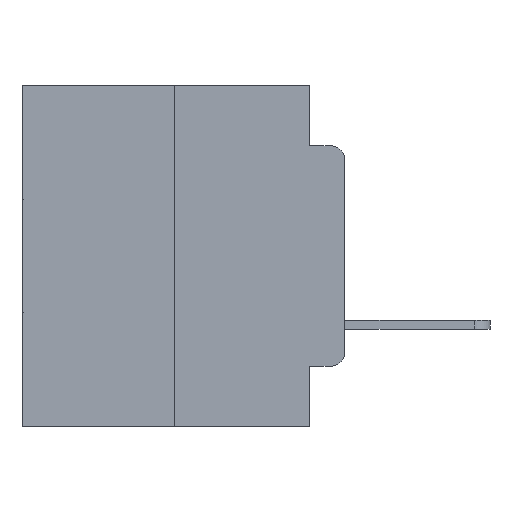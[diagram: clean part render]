
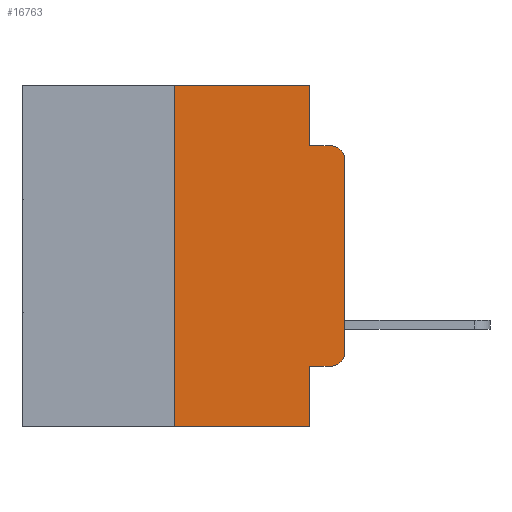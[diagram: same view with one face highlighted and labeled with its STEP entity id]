
A CAD part, left-side view. The second image highlights one B-rep face of the part: STEP entity #16763.
In plain terms, the highlighted planar face has unit normal (-1, 0, 0).
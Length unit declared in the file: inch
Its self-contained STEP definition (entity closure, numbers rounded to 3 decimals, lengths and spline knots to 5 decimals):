
#616 = DIRECTION ( 'NONE',  ( 1., 0., 0. ) ) ;
#1501 = DIRECTION ( 'NONE',  ( 0., 0., -1. ) ) ;
#1969 = VERTEX_POINT ( 'NONE', #9415 ) ;
#2576 = CARTESIAN_POINT ( 'NONE',  ( 0., 0., -0.1085 ) ) ;
#2963 = CARTESIAN_POINT ( 'NONE',  ( 0., 0.473, 0. ) ) ;
#3469 = VERTEX_POINT ( 'NONE', #17438 ) ;
#4350 = DIRECTION ( 'NONE',  ( 0., 0., 1. ) ) ;
#4463 = DIRECTION ( 'NONE',  ( 0., 0., 1. ) ) ;
#5062 = EDGE_CURVE ( 'NONE', #19786, #3469, #8488, .T. ) ;
#5736 = ORIENTED_EDGE ( 'NONE', *, *, #23668, .T. ) ;
#6091 = VECTOR ( 'NONE', #17724, 39.37008 ) ;
#6179 = EDGE_CURVE ( 'NONE', #1969, #26335, #27511, .T. ) ;
#6511 = DIRECTION ( 'NONE',  ( 0., -1., 0. ) ) ;
#6670 = VECTOR ( 'NONE', #14076, 39.37008 ) ;
#6709 = CARTESIAN_POINT ( 'NONE',  ( 0., 0.25, 0. ) ) ;
#6812 = LINE ( 'NONE', #9000, #6091 ) ;
#6977 = CARTESIAN_POINT ( 'NONE',  ( 0., 0., -0.3915 ) ) ;
#7083 = CARTESIAN_POINT ( 'NONE',  ( 0., 0.25, -0.5 ) ) ;
#7848 = ORIENTED_EDGE ( 'NONE', *, *, #14998, .F. ) ;
#7859 = CARTESIAN_POINT ( 'NONE',  ( 0., 0.051, 0. ) ) ;
#8178 = ORIENTED_EDGE ( 'NONE', *, *, #5062, .T. ) ;
#8261 = CARTESIAN_POINT ( 'NONE',  ( 0., 0.473, 0. ) ) ;
#8488 = LINE ( 'NONE', #9616, #19468 ) ;
#8993 = CIRCLE ( 'NONE', #9815, 0.02 ) ;
#9000 = CARTESIAN_POINT ( 'NONE',  ( 0., 0.051, -0.4115 ) ) ;
#9369 = DIRECTION ( 'NONE',  ( -1., 0., 0. ) ) ;
#9415 = CARTESIAN_POINT ( 'NONE',  ( 0., 0.02, -0.4115 ) ) ;
#9616 = CARTESIAN_POINT ( 'NONE',  ( 0., 0.473, -0.5 ) ) ;
#9722 = LINE ( 'NONE', #6709, #14796 ) ;
#9815 = AXIS2_PLACEMENT_3D ( 'NONE', #22352, #9369, #24483 ) ;
#9846 = CARTESIAN_POINT ( 'NONE',  ( 0., 0.051, 0. ) ) ;
#9970 = LINE ( 'NONE', #16199, #16475 ) ;
#10102 = VERTEX_POINT ( 'NONE', #2576 ) ;
#10635 = EDGE_CURVE ( 'NONE', #17381, #1969, #6812, .T. ) ;
#10940 = CARTESIAN_POINT ( 'NONE',  ( 0., 0., 0. ) ) ;
#11875 = LINE ( 'NONE', #21744, #23367 ) ;
#11917 = EDGE_LOOP ( 'NONE', ( #5736, #28208, #18121, #7848, #12577, #22993, #8178, #25340, #24726, #13520 ) ) ;
#12064 = EDGE_CURVE ( 'NONE', #17381, #3469, #23996, .T. ) ;
#12106 = LINE ( 'NONE', #8261, #24026 ) ;
#12302 = VERTEX_POINT ( 'NONE', #25534 ) ;
#12342 = AXIS2_PLACEMENT_3D ( 'NONE', #2963, #616, #16387 ) ;
#12577 = ORIENTED_EDGE ( 'NONE', *, *, #22984, .F. ) ;
#13462 = EDGE_CURVE ( 'NONE', #19786, #12302, #9722, .T. ) ;
#13520 = ORIENTED_EDGE ( 'NONE', *, *, #6179, .T. ) ;
#13897 = DIRECTION ( 'NONE',  ( 0., 0., -1. ) ) ;
#14076 = DIRECTION ( 'NONE',  ( 0., 0., -1. ) ) ;
#14358 = CARTESIAN_POINT ( 'NONE',  ( 0., 0.051, -0.4115 ) ) ;
#14796 = VECTOR ( 'NONE', #4463, 39.37008 ) ;
#14917 = DIRECTION ( 'NONE',  ( -1., 0., 0. ) ) ;
#14998 = EDGE_CURVE ( 'NONE', #16822, #21267, #9970, .T. ) ;
#16199 = CARTESIAN_POINT ( 'NONE',  ( 0., 0.051, 0. ) ) ;
#16221 = DIRECTION ( 'NONE',  ( 0., -1., 0. ) ) ;
#16387 = DIRECTION ( 'NONE',  ( 0., 0., -1. ) ) ;
#16475 = VECTOR ( 'NONE', #13897, 39.37008 ) ;
#16500 = EDGE_CURVE ( 'NONE', #21267, #26684, #11875, .T. ) ;
#16763 = ADVANCED_FACE ( 'NONE', ( #21696 ), #22761, .F. ) ;
#16822 = VERTEX_POINT ( 'NONE', #7859 ) ;
#16892 = VECTOR ( 'NONE', #4350, 39.37008 ) ;
#17381 = VERTEX_POINT ( 'NONE', #14358 ) ;
#17438 = CARTESIAN_POINT ( 'NONE',  ( 0., 0.051, -0.5 ) ) ;
#17724 = DIRECTION ( 'NONE',  ( 0., -1., 0. ) ) ;
#18121 = ORIENTED_EDGE ( 'NONE', *, *, #16500, .F. ) ;
#19468 = VECTOR ( 'NONE', #16221, 39.37008 ) ;
#19786 = VERTEX_POINT ( 'NONE', #7083 ) ;
#19824 = AXIS2_PLACEMENT_3D ( 'NONE', #27599, #14917, #1501 ) ;
#21267 = VERTEX_POINT ( 'NONE', #21874 ) ;
#21696 = FACE_OUTER_BOUND ( 'NONE', #11917, .T. ) ;
#21744 = CARTESIAN_POINT ( 'NONE',  ( 0., 0.051, -0.0885 ) ) ;
#21874 = CARTESIAN_POINT ( 'NONE',  ( 0., 0.051, -0.0885 ) ) ;
#22251 = EDGE_CURVE ( 'NONE', #10102, #26684, #8993, .T. ) ;
#22352 = CARTESIAN_POINT ( 'NONE',  ( 0., 0.02, -0.1085 ) ) ;
#22593 = LINE ( 'NONE', #10940, #16892 ) ;
#22761 = PLANE ( 'NONE',  #12342 ) ;
#22984 = EDGE_CURVE ( 'NONE', #12302, #16822, #12106, .T. ) ;
#22993 = ORIENTED_EDGE ( 'NONE', *, *, #13462, .F. ) ;
#23367 = VECTOR ( 'NONE', #6511, 39.37008 ) ;
#23668 = EDGE_CURVE ( 'NONE', #26335, #10102, #22593, .T. ) ;
#23996 = LINE ( 'NONE', #9846, #6670 ) ;
#24026 = VECTOR ( 'NONE', #25510, 39.37008 ) ;
#24483 = DIRECTION ( 'NONE',  ( 0., 0., -1. ) ) ;
#24726 = ORIENTED_EDGE ( 'NONE', *, *, #10635, .T. ) ;
#25340 = ORIENTED_EDGE ( 'NONE', *, *, #12064, .F. ) ;
#25510 = DIRECTION ( 'NONE',  ( 0., -1., 0. ) ) ;
#25534 = CARTESIAN_POINT ( 'NONE',  ( 0., 0.25, 0. ) ) ;
#26335 = VERTEX_POINT ( 'NONE', #6977 ) ;
#26684 = VERTEX_POINT ( 'NONE', #27306 ) ;
#27306 = CARTESIAN_POINT ( 'NONE',  ( 0., 0.02, -0.0885 ) ) ;
#27511 = CIRCLE ( 'NONE', #19824, 0.02 ) ;
#27599 = CARTESIAN_POINT ( 'NONE',  ( 0., 0.02, -0.3915 ) ) ;
#28208 = ORIENTED_EDGE ( 'NONE', *, *, #22251, .T. ) ;
